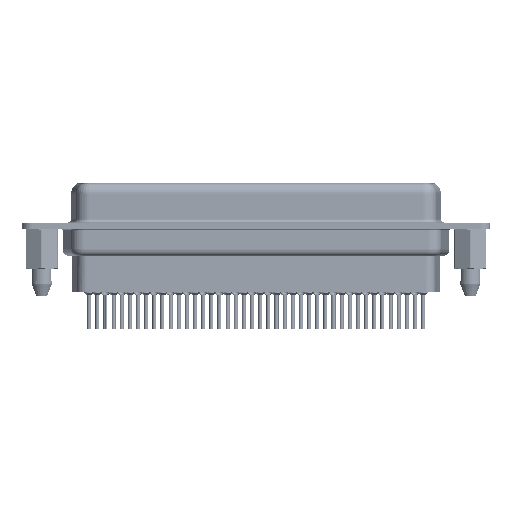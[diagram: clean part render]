
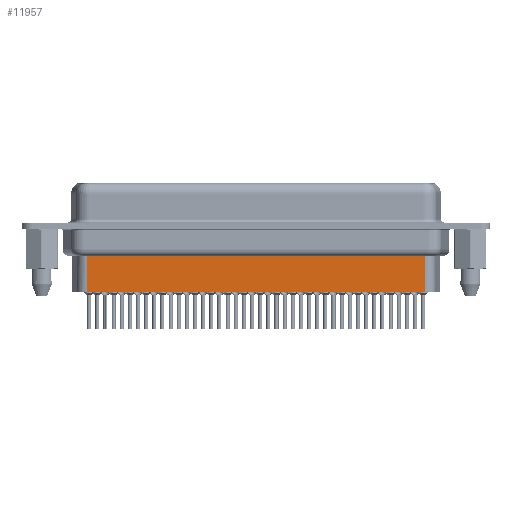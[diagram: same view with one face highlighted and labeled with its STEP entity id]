
A CAD part, front view. The second image highlights one B-rep face of the part: STEP entity #11957.
In plain terms, the highlighted planar face has unit normal (0, -1, 0).
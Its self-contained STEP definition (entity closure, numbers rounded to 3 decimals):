
#3455 = LINE ( 'NONE', #10778, #33728 ) ;
#4192 = CARTESIAN_POINT ( 'NONE',  ( 6.706, -3.5, -3.1 ) ) ;
#6855 = EDGE_CURVE ( 'NONE', #44195, #16104, #19690, .T. ) ;
#7178 = ORIENTED_EDGE ( 'NONE', *, *, #28316, .F. ) ;
#8097 = DIRECTION ( 'NONE',  ( 1., 0., 0. ) ) ;
#8383 = ORIENTED_EDGE ( 'NONE', *, *, #6855, .F. ) ;
#10190 = DIRECTION ( 'NONE',  ( -1., 0., 0. ) ) ;
#10302 = ORIENTED_EDGE ( 'NONE', *, *, #36673, .T. ) ;
#10778 = CARTESIAN_POINT ( 'NONE',  ( 6.706, -3.5, -3.1 ) ) ;
#11515 = FACE_OUTER_BOUND ( 'NONE', #41113, .T. ) ;
#11957 = ADVANCED_FACE ( 'NONE', ( #11515 ), #41469, .T. ) ;
#15878 = EDGE_CURVE ( 'NONE', #29069, #33697, #3455, .T. ) ;
#16104 = VERTEX_POINT ( 'NONE', #25288 ) ;
#16346 = CARTESIAN_POINT ( 'NONE',  ( 6.706, -3.5, -4.097 ) ) ;
#19690 = LINE ( 'NONE', #45770, #30850 ) ;
#20669 = VECTOR ( 'NONE', #10190, 1000. ) ;
#22249 = CARTESIAN_POINT ( 'NONE',  ( 6.706, -3.5, -9.85 ) ) ;
#22956 = DIRECTION ( 'NONE',  ( -1., 0., 0. ) ) ;
#25288 = CARTESIAN_POINT ( 'NONE',  ( 56.794, -3.5, -9.85 ) ) ;
#26636 = CARTESIAN_POINT ( 'NONE',  ( 6.459, -3.5, -4.097 ) ) ;
#28316 = EDGE_CURVE ( 'NONE', #16104, #33697, #32087, .T. ) ;
#29069 = VERTEX_POINT ( 'NONE', #16346 ) ;
#30850 = VECTOR ( 'NONE', #31859, 1000. ) ;
#31859 = DIRECTION ( 'NONE',  ( 0., 0., -1. ) ) ;
#32087 = LINE ( 'NONE', #22249, #20669 ) ;
#33155 = DIRECTION ( 'NONE',  ( 0., 0., -1. ) ) ;
#33186 = LINE ( 'NONE', #26636, #45234 ) ;
#33697 = VERTEX_POINT ( 'NONE', #43996 ) ;
#33728 = VECTOR ( 'NONE', #33155, 1000. ) ;
#33888 = DIRECTION ( 'NONE',  ( 0., -1., 0. ) ) ;
#35801 = AXIS2_PLACEMENT_3D ( 'NONE', #4192, #33888, #8097 ) ;
#36673 = EDGE_CURVE ( 'NONE', #44195, #29069, #33186, .T. ) ;
#37697 = ORIENTED_EDGE ( 'NONE', *, *, #15878, .T. ) ;
#41113 = EDGE_LOOP ( 'NONE', ( #8383, #10302, #37697, #7178 ) ) ;
#41469 = PLANE ( 'NONE',  #35801 ) ;
#42498 = CARTESIAN_POINT ( 'NONE',  ( 56.794, -3.5, -4.097 ) ) ;
#43996 = CARTESIAN_POINT ( 'NONE',  ( 6.706, -3.5, -9.85 ) ) ;
#44195 = VERTEX_POINT ( 'NONE', #42498 ) ;
#45234 = VECTOR ( 'NONE', #22956, 1000. ) ;
#45770 = CARTESIAN_POINT ( 'NONE',  ( 56.794, -3.5, -3.1 ) ) ;
